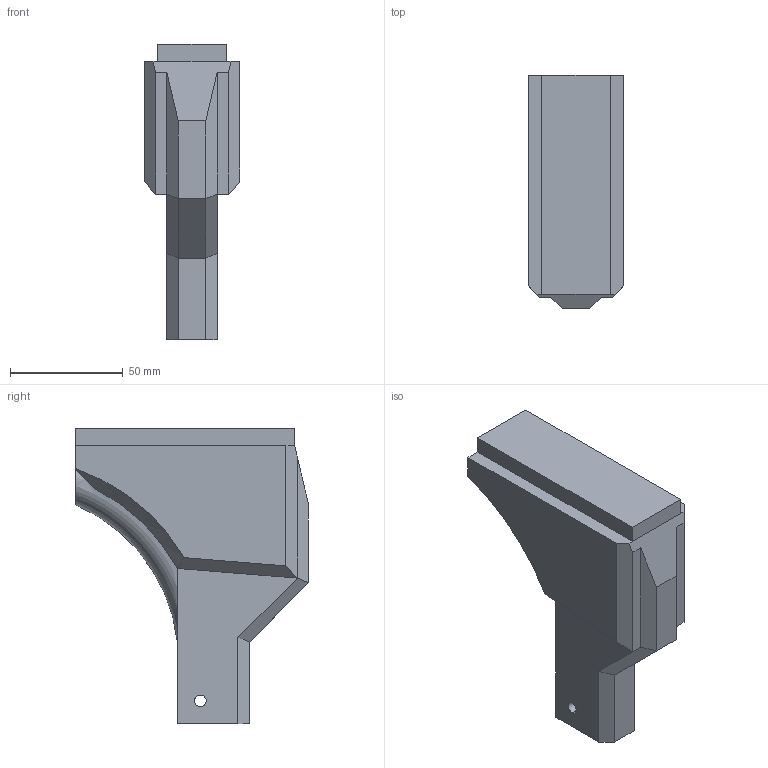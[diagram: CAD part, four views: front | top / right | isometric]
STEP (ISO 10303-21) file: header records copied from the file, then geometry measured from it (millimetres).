
FILE_DESCRIPTION (( 'STEP AP214' ), '1' );
FILE_NAME ('hydrastocky1.STEP', '2013-07-04T02:35:39', ( '' ), ( '' ), 'SwSTEP 2.0', 'SolidWorks 2012', '' );
FILE_SCHEMA (( 'AUTOMOTIVE_DESIGN' ));
Length unit declared in the file: millimetre
Products named in the file (1): hydrastocky1
Bounding box: 42.24 x 103.11 x 130.92 mm (x, y, z)
Volume: 267719.7 mm3; surface area: 31150.5 mm2
Topology: 1 solids, 1 shells, 53 faces, 137 edges, 86 vertices
Faces by surface type: plane 42, cylinder 7, torus 2, cone 2
Entity records: 1753 total; most frequent: CARTESIAN_POINT 431, ORIENTED_EDGE 274, DIRECTION 251, EDGE_CURVE 137, VECTOR 107, LINE 107, VERTEX_POINT 86, AXIS2_PLACEMENT_3D 72
